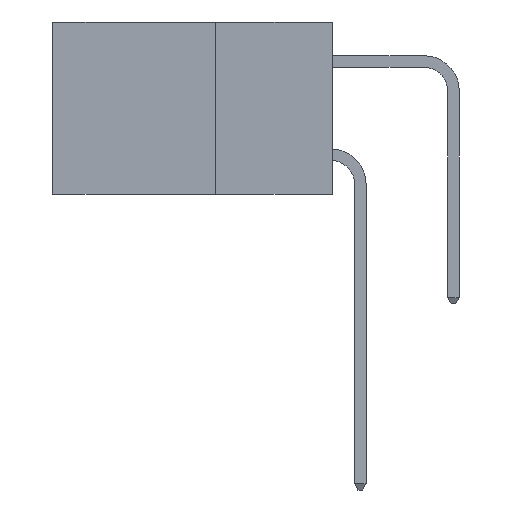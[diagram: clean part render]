
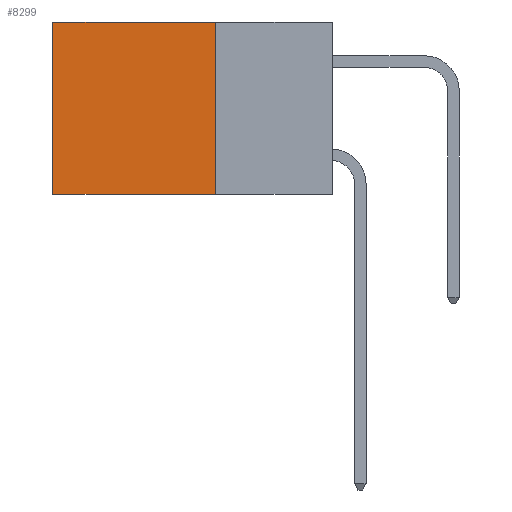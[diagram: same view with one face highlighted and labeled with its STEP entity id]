
A CAD part, left-side view. The second image highlights one B-rep face of the part: STEP entity #8299.
In plain terms, the highlighted planar face has unit normal (-1, 0, 0).
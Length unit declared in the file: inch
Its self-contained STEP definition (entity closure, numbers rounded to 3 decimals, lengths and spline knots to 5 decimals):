
#705 = EDGE_CURVE ( 'NONE', #1350, #1026, #12204, .T. ) ;
#842 = DIRECTION ( 'NONE',  ( 0., 1., 0. ) ) ;
#939 = LINE ( 'NONE', #1640, #7402 ) ;
#1010 = FACE_OUTER_BOUND ( 'NONE', #13004, .T. ) ;
#1026 = VERTEX_POINT ( 'NONE', #7081 ) ;
#1350 = VERTEX_POINT ( 'NONE', #11058 ) ;
#1511 = CARTESIAN_POINT ( 'NONE',  ( 0.2615, 0.25, 0. ) ) ;
#1606 = DIRECTION ( 'NONE',  ( 0., 0., -1. ) ) ;
#1640 = CARTESIAN_POINT ( 'NONE',  ( 0.2615, 0.6, -0.37 ) ) ;
#1762 = VECTOR ( 'NONE', #842, 39.37008 ) ;
#2410 = DIRECTION ( 'NONE',  ( 0., 0., -1. ) ) ;
#2454 = DIRECTION ( 'NONE',  ( 1., 0., 0. ) ) ;
#2633 = CARTESIAN_POINT ( 'NONE',  ( 0.2615, 0.25, -0.37 ) ) ;
#2741 = PLANE ( 'NONE',  #11250 ) ;
#3106 = DIRECTION ( 'NONE',  ( 0., 0., -1. ) ) ;
#3261 = CARTESIAN_POINT ( 'NONE',  ( 0.2615, 0.25, -0.37 ) ) ;
#3715 = EDGE_CURVE ( 'NONE', #14393, #8981, #939, .T. ) ;
#4125 = EDGE_CURVE ( 'NONE', #1350, #14393, #14667, .T. ) ;
#5065 = LINE ( 'NONE', #14163, #14955 ) ;
#7081 = CARTESIAN_POINT ( 'NONE',  ( 0.2615, 0.25, -0.37 ) ) ;
#7402 = VECTOR ( 'NONE', #1606, 39.37008 ) ;
#8230 = ORIENTED_EDGE ( 'NONE', *, *, #3715, .T. ) ;
#8299 = ADVANCED_FACE ( 'NONE', ( #1010 ), #2741, .F. ) ;
#8915 = ORIENTED_EDGE ( 'NONE', *, *, #705, .F. ) ;
#8981 = VERTEX_POINT ( 'NONE', #12918 ) ;
#11058 = CARTESIAN_POINT ( 'NONE',  ( 0.2615, 0.25, 0. ) ) ;
#11250 = AXIS2_PLACEMENT_3D ( 'NONE', #2633, #2454, #2410 ) ;
#12204 = LINE ( 'NONE', #3261, #12602 ) ;
#12602 = VECTOR ( 'NONE', #3106, 39.37008 ) ;
#12918 = CARTESIAN_POINT ( 'NONE',  ( 0.2615, 0.6, -0.37 ) ) ;
#12962 = ORIENTED_EDGE ( 'NONE', *, *, #15656, .F. ) ;
#13004 = EDGE_LOOP ( 'NONE', ( #8230, #12962, #8915, #15047 ) ) ;
#14163 = CARTESIAN_POINT ( 'NONE',  ( 0.2615, 0.25, -0.37 ) ) ;
#14393 = VERTEX_POINT ( 'NONE', #15579 ) ;
#14667 = LINE ( 'NONE', #1511, #1762 ) ;
#14955 = VECTOR ( 'NONE', #15441, 39.37008 ) ;
#15047 = ORIENTED_EDGE ( 'NONE', *, *, #4125, .T. ) ;
#15441 = DIRECTION ( 'NONE',  ( 0., 1., 0. ) ) ;
#15579 = CARTESIAN_POINT ( 'NONE',  ( 0.2615, 0.6, 0. ) ) ;
#15656 = EDGE_CURVE ( 'NONE', #1026, #8981, #5065, .T. ) ;
